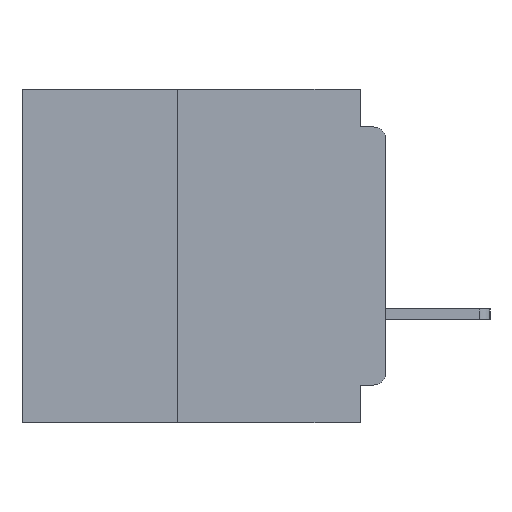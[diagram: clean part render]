
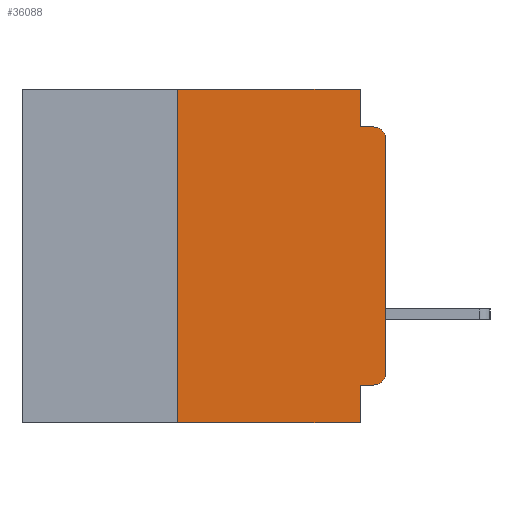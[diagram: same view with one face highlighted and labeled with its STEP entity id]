
A CAD part, left-side view. The second image highlights one B-rep face of the part: STEP entity #36088.
In plain terms, the highlighted planar face has unit normal (-1, 0, 0).
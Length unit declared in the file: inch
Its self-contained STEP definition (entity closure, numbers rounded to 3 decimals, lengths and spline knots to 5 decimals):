
#132 = VERTEX_POINT ( 'NONE', #41087 ) ;
#389 = CARTESIAN_POINT ( 'NONE',  ( 0., 0.031, 0. ) ) ;
#505 = CARTESIAN_POINT ( 'NONE',  ( 0., 0., -0.06 ) ) ;
#1448 = VERTEX_POINT ( 'NONE', #34289 ) ;
#1449 = VERTEX_POINT ( 'NONE', #505 ) ;
#2242 = DIRECTION ( 'NONE',  ( 1., 0., 0. ) ) ;
#2775 = VERTEX_POINT ( 'NONE', #29458 ) ;
#3026 = LINE ( 'NONE', #13746, #20190 ) ;
#3801 = CARTESIAN_POINT ( 'NONE',  ( 0., 0., 0. ) ) ;
#3820 = VECTOR ( 'NONE', #31273, 39.37008 ) ;
#3910 = ORIENTED_EDGE ( 'NONE', *, *, #13895, .T. ) ;
#3957 = ORIENTED_EDGE ( 'NONE', *, *, #6639, .F. ) ;
#3980 = CARTESIAN_POINT ( 'NONE',  ( 0., 0., -0.355 ) ) ;
#4477 = ORIENTED_EDGE ( 'NONE', *, *, #39385, .F. ) ;
#5142 = ORIENTED_EDGE ( 'NONE', *, *, #33604, .F. ) ;
#5237 = CARTESIAN_POINT ( 'NONE',  ( 0., 0.015, -0.045 ) ) ;
#6246 = AXIS2_PLACEMENT_3D ( 'NONE', #16515, #40291, #19965 ) ;
#6487 = DIRECTION ( 'NONE',  ( 0., -1., 0. ) ) ;
#6609 = ORIENTED_EDGE ( 'NONE', *, *, #18807, .F. ) ;
#6639 = EDGE_CURVE ( 'NONE', #1448, #8491, #25710, .T. ) ;
#6752 = ORIENTED_EDGE ( 'NONE', *, *, #24700, .F. ) ;
#7428 = EDGE_CURVE ( 'NONE', #9873, #132, #17640, .T. ) ;
#8262 = LINE ( 'NONE', #32787, #42297 ) ;
#8423 = VERTEX_POINT ( 'NONE', #15087 ) ;
#8491 = VERTEX_POINT ( 'NONE', #5237 ) ;
#9873 = VERTEX_POINT ( 'NONE', #16544 ) ;
#11518 = CARTESIAN_POINT ( 'NONE',  ( 0., 0., -0.045 ) ) ;
#12458 = CARTESIAN_POINT ( 'NONE',  ( 0., 0.437, 0. ) ) ;
#13445 = CARTESIAN_POINT ( 'NONE',  ( 0., 0.031, 0. ) ) ;
#13686 = CARTESIAN_POINT ( 'NONE',  ( 0., 0.031, -0.355 ) ) ;
#13746 = CARTESIAN_POINT ( 'NONE',  ( 0., 0.437, 0. ) ) ;
#13895 = EDGE_CURVE ( 'NONE', #132, #1449, #40576, .T. ) ;
#14188 = VECTOR ( 'NONE', #6487, 39.37008 ) ;
#14737 = DIRECTION ( 'NONE',  ( -1., 0., 0. ) ) ;
#14786 = VERTEX_POINT ( 'NONE', #13686 ) ;
#15087 = CARTESIAN_POINT ( 'NONE',  ( 0., 0.25, -0.4 ) ) ;
#15135 = VECTOR ( 'NONE', #22314, 39.37008 ) ;
#16052 = AXIS2_PLACEMENT_3D ( 'NONE', #12458, #2242, #26177 ) ;
#16515 = CARTESIAN_POINT ( 'NONE',  ( 0., 0.015, -0.34 ) ) ;
#16544 = CARTESIAN_POINT ( 'NONE',  ( 0., 0.015, -0.355 ) ) ;
#16879 = DIRECTION ( 'NONE',  ( 0., 0., -1. ) ) ;
#17640 = CIRCLE ( 'NONE', #6246, 0.015 ) ;
#18007 = LINE ( 'NONE', #13445, #25989 ) ;
#18807 = EDGE_CURVE ( 'NONE', #21567, #1448, #18007, .T. ) ;
#19283 = DIRECTION ( 'NONE',  ( 0., 0., -1. ) ) ;
#19965 = DIRECTION ( 'NONE',  ( 0., 0., -1. ) ) ;
#20190 = VECTOR ( 'NONE', #34131, 39.37008 ) ;
#21567 = VERTEX_POINT ( 'NONE', #389 ) ;
#21684 = ORIENTED_EDGE ( 'NONE', *, *, #40563, .T. ) ;
#21821 = CIRCLE ( 'NONE', #41057, 0.015 ) ;
#22314 = DIRECTION ( 'NONE',  ( 0., 0., 1. ) ) ;
#22743 = PLANE ( 'NONE',  #16052 ) ;
#23068 = LINE ( 'NONE', #3980, #3820 ) ;
#24200 = LINE ( 'NONE', #42648, #15135 ) ;
#24700 = EDGE_CURVE ( 'NONE', #14786, #2775, #8262, .T. ) ;
#25415 = LINE ( 'NONE', #30296, #14188 ) ;
#25710 = LINE ( 'NONE', #11518, #41637 ) ;
#25989 = VECTOR ( 'NONE', #16879, 39.37008 ) ;
#26177 = DIRECTION ( 'NONE',  ( 0., 0., -1. ) ) ;
#27686 = DIRECTION ( 'NONE',  ( 0., 0., 1. ) ) ;
#27741 = EDGE_CURVE ( 'NONE', #1449, #8491, #21821, .T. ) ;
#29458 = CARTESIAN_POINT ( 'NONE',  ( 0., 0.031, -0.4 ) ) ;
#29614 = VERTEX_POINT ( 'NONE', #40117 ) ;
#29685 = ORIENTED_EDGE ( 'NONE', *, *, #7428, .T. ) ;
#30296 = CARTESIAN_POINT ( 'NONE',  ( 0., 0.437, -0.4 ) ) ;
#30457 = VECTOR ( 'NONE', #27686, 39.37008 ) ;
#31273 = DIRECTION ( 'NONE',  ( 0., 1., 0. ) ) ;
#32787 = CARTESIAN_POINT ( 'NONE',  ( 0., 0.031, -0.4 ) ) ;
#33264 = FACE_OUTER_BOUND ( 'NONE', #36132, .T. ) ;
#33604 = EDGE_CURVE ( 'NONE', #9873, #14786, #23068, .T. ) ;
#34131 = DIRECTION ( 'NONE',  ( 0., -1., 0. ) ) ;
#34289 = CARTESIAN_POINT ( 'NONE',  ( 0., 0.031, -0.045 ) ) ;
#35122 = CARTESIAN_POINT ( 'NONE',  ( 0., 0.015, -0.06 ) ) ;
#36088 = ADVANCED_FACE ( 'NONE', ( #33264 ), #22743, .F. ) ;
#36132 = EDGE_LOOP ( 'NONE', ( #3910, #39661, #3957, #6609, #4477, #41791, #21684, #6752, #5142, #29685 ) ) ;
#38517 = DIRECTION ( 'NONE',  ( 0., 0., -1. ) ) ;
#38714 = DIRECTION ( 'NONE',  ( 0., -1., 0. ) ) ;
#39385 = EDGE_CURVE ( 'NONE', #29614, #21567, #3026, .T. ) ;
#39661 = ORIENTED_EDGE ( 'NONE', *, *, #27741, .T. ) ;
#40117 = CARTESIAN_POINT ( 'NONE',  ( 0., 0.25, 0. ) ) ;
#40291 = DIRECTION ( 'NONE',  ( -1., 0., 0. ) ) ;
#40563 = EDGE_CURVE ( 'NONE', #8423, #2775, #25415, .T. ) ;
#40576 = LINE ( 'NONE', #3801, #30457 ) ;
#41057 = AXIS2_PLACEMENT_3D ( 'NONE', #35122, #14737, #38517 ) ;
#41087 = CARTESIAN_POINT ( 'NONE',  ( 0., 0., -0.34 ) ) ;
#41637 = VECTOR ( 'NONE', #38714, 39.37008 ) ;
#41791 = ORIENTED_EDGE ( 'NONE', *, *, #42192, .F. ) ;
#42192 = EDGE_CURVE ( 'NONE', #8423, #29614, #24200, .T. ) ;
#42297 = VECTOR ( 'NONE', #19283, 39.37008 ) ;
#42648 = CARTESIAN_POINT ( 'NONE',  ( 0., 0.25, -0.4 ) ) ;
